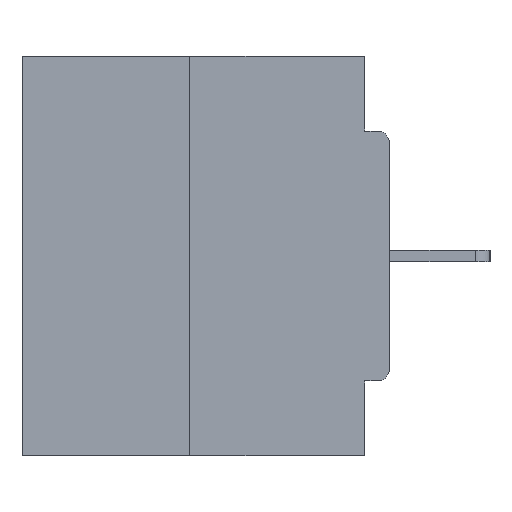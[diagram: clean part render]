
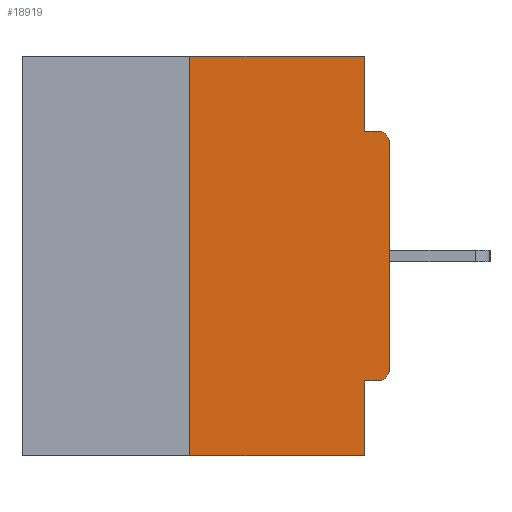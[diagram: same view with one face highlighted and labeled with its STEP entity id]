
A CAD part, left-side view. The second image highlights one B-rep face of the part: STEP entity #18919.
In plain terms, the highlighted planar face has unit normal (-1, 0, 0).
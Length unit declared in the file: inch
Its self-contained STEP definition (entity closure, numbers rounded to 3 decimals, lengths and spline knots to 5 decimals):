
#162 = CARTESIAN_POINT ( 'NONE',  ( 0., 0.25, 0. ) ) ;
#612 = CARTESIAN_POINT ( 'NONE',  ( 0., 0., 0. ) ) ;
#1217 = EDGE_CURVE ( 'NONE', #28843, #24404, #7642, .T. ) ;
#1417 = DIRECTION ( 'NONE',  ( 1., 0., 0. ) ) ;
#2264 = VERTEX_POINT ( 'NONE', #15875 ) ;
#2714 = LINE ( 'NONE', #16824, #29427 ) ;
#2733 = DIRECTION ( 'NONE',  ( 0., -1., 0. ) ) ;
#3099 = DIRECTION ( 'NONE',  ( 0., 0., 1. ) ) ;
#3276 = CARTESIAN_POINT ( 'NONE',  ( 0., 0.46, 0. ) ) ;
#3893 = PLANE ( 'NONE',  #12326 ) ;
#4582 = ORIENTED_EDGE ( 'NONE', *, *, #5427, .F. ) ;
#5427 = EDGE_CURVE ( 'NONE', #23310, #2264, #2714, .T. ) ;
#5599 = LINE ( 'NONE', #12719, #21315 ) ;
#6086 = CARTESIAN_POINT ( 'NONE',  ( 0., 0.031, -0.5 ) ) ;
#6368 = VERTEX_POINT ( 'NONE', #162 ) ;
#6713 = AXIS2_PLACEMENT_3D ( 'NONE', #12950, #25006, #32470 ) ;
#7282 = EDGE_CURVE ( 'NONE', #20162, #2264, #21503, .T. ) ;
#7442 = CARTESIAN_POINT ( 'NONE',  ( 0., 0., -0.3915 ) ) ;
#7533 = CARTESIAN_POINT ( 'NONE',  ( 0., 0.46, -0.5 ) ) ;
#7642 = CIRCLE ( 'NONE', #8699, 0.015 ) ;
#7673 = DIRECTION ( 'NONE',  ( 0., -1., 0. ) ) ;
#8414 = VERTEX_POINT ( 'NONE', #16319 ) ;
#8475 = VECTOR ( 'NONE', #13372, 39.37008 ) ;
#8699 = AXIS2_PLACEMENT_3D ( 'NONE', #12363, #29438, #12523 ) ;
#10396 = ORIENTED_EDGE ( 'NONE', *, *, #7282, .T. ) ;
#11514 = DIRECTION ( 'NONE',  ( 0., 0., -1. ) ) ;
#11624 = ORIENTED_EDGE ( 'NONE', *, *, #21552, .F. ) ;
#12044 = DIRECTION ( 'NONE',  ( 0., 0., 1. ) ) ;
#12326 = AXIS2_PLACEMENT_3D ( 'NONE', #13985, #1417, #11514 ) ;
#12363 = CARTESIAN_POINT ( 'NONE',  ( 0., 0.015, -0.3915 ) ) ;
#12476 = DIRECTION ( 'NONE',  ( 0., 0., -1. ) ) ;
#12523 = DIRECTION ( 'NONE',  ( 0., 0., -1. ) ) ;
#12719 = CARTESIAN_POINT ( 'NONE',  ( 0., 0.031, 0. ) ) ;
#12855 = VECTOR ( 'NONE', #3099, 39.37008 ) ;
#12950 = CARTESIAN_POINT ( 'NONE',  ( 0., 0.015, -0.1085 ) ) ;
#13221 = CARTESIAN_POINT ( 'NONE',  ( 0., 0.015, -0.4065 ) ) ;
#13372 = DIRECTION ( 'NONE',  ( 0., -1., 0. ) ) ;
#13501 = EDGE_CURVE ( 'NONE', #6368, #18191, #15187, .T. ) ;
#13908 = ORIENTED_EDGE ( 'NONE', *, *, #24772, .F. ) ;
#13985 = CARTESIAN_POINT ( 'NONE',  ( 0., 0.46, 0. ) ) ;
#14019 = CARTESIAN_POINT ( 'NONE',  ( 0., 0.031, -0.0935 ) ) ;
#14288 = VECTOR ( 'NONE', #18112, 39.37008 ) ;
#15187 = LINE ( 'NONE', #3276, #8475 ) ;
#15875 = CARTESIAN_POINT ( 'NONE',  ( 0., 0.015, -0.0935 ) ) ;
#16059 = VECTOR ( 'NONE', #2733, 39.37008 ) ;
#16319 = CARTESIAN_POINT ( 'NONE',  ( 0., 0.031, -0.4065 ) ) ;
#16375 = ORIENTED_EDGE ( 'NONE', *, *, #25998, .T. ) ;
#16824 = CARTESIAN_POINT ( 'NONE',  ( 0., 0., -0.0935 ) ) ;
#17349 = LINE ( 'NONE', #20601, #14288 ) ;
#17603 = EDGE_CURVE ( 'NONE', #8414, #23372, #25540, .T. ) ;
#18112 = DIRECTION ( 'NONE',  ( 0., 1., 0. ) ) ;
#18191 = VERTEX_POINT ( 'NONE', #21193 ) ;
#18919 = ADVANCED_FACE ( 'NONE', ( #26550 ), #3893, .F. ) ;
#19154 = EDGE_CURVE ( 'NONE', #25122, #23372, #25379, .T. ) ;
#19484 = CARTESIAN_POINT ( 'NONE',  ( 0., 0.25, 0. ) ) ;
#20162 = VERTEX_POINT ( 'NONE', #21932 ) ;
#20601 = CARTESIAN_POINT ( 'NONE',  ( 0., 0., -0.4065 ) ) ;
#21193 = CARTESIAN_POINT ( 'NONE',  ( 0., 0.031, 0. ) ) ;
#21315 = VECTOR ( 'NONE', #30404, 39.37008 ) ;
#21503 = CIRCLE ( 'NONE', #6713, 0.015 ) ;
#21552 = EDGE_CURVE ( 'NONE', #28843, #8414, #17349, .T. ) ;
#21932 = CARTESIAN_POINT ( 'NONE',  ( 0., 0., -0.1085 ) ) ;
#22410 = CARTESIAN_POINT ( 'NONE',  ( 0., 0.031, -0.5 ) ) ;
#23310 = VERTEX_POINT ( 'NONE', #14019 ) ;
#23372 = VERTEX_POINT ( 'NONE', #6086 ) ;
#24241 = CARTESIAN_POINT ( 'NONE',  ( 0., 0.25, -0.5 ) ) ;
#24404 = VERTEX_POINT ( 'NONE', #7442 ) ;
#24772 = EDGE_CURVE ( 'NONE', #25122, #6368, #26927, .T. ) ;
#25006 = DIRECTION ( 'NONE',  ( -1., 0., 0. ) ) ;
#25122 = VERTEX_POINT ( 'NONE', #24241 ) ;
#25379 = LINE ( 'NONE', #7533, #16059 ) ;
#25540 = LINE ( 'NONE', #22410, #30753 ) ;
#25998 = EDGE_CURVE ( 'NONE', #24404, #20162, #30223, .T. ) ;
#26016 = VECTOR ( 'NONE', #12044, 39.37008 ) ;
#26550 = FACE_OUTER_BOUND ( 'NONE', #27720, .T. ) ;
#26826 = ORIENTED_EDGE ( 'NONE', *, *, #17603, .F. ) ;
#26927 = LINE ( 'NONE', #19484, #26016 ) ;
#27502 = EDGE_CURVE ( 'NONE', #18191, #23310, #5599, .T. ) ;
#27626 = ORIENTED_EDGE ( 'NONE', *, *, #13501, .F. ) ;
#27720 = EDGE_LOOP ( 'NONE', ( #27626, #13908, #32070, #26826, #11624, #30398, #16375, #10396, #4582, #31118 ) ) ;
#28843 = VERTEX_POINT ( 'NONE', #13221 ) ;
#29427 = VECTOR ( 'NONE', #7673, 39.37008 ) ;
#29438 = DIRECTION ( 'NONE',  ( -1., 0., 0. ) ) ;
#30223 = LINE ( 'NONE', #612, #12855 ) ;
#30398 = ORIENTED_EDGE ( 'NONE', *, *, #1217, .T. ) ;
#30404 = DIRECTION ( 'NONE',  ( 0., 0., -1. ) ) ;
#30753 = VECTOR ( 'NONE', #12476, 39.37008 ) ;
#31118 = ORIENTED_EDGE ( 'NONE', *, *, #27502, .F. ) ;
#32070 = ORIENTED_EDGE ( 'NONE', *, *, #19154, .T. ) ;
#32470 = DIRECTION ( 'NONE',  ( 0., 0., -1. ) ) ;
